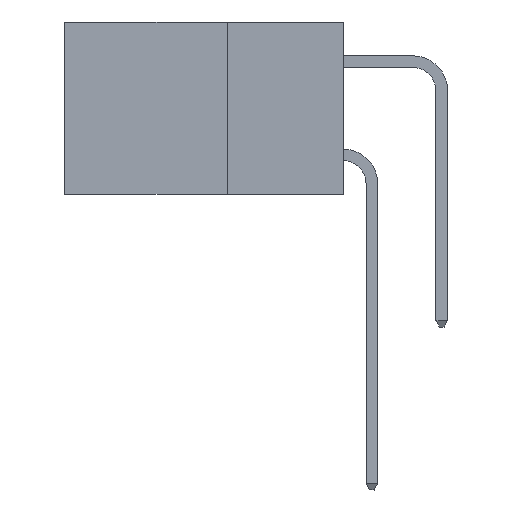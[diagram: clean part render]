
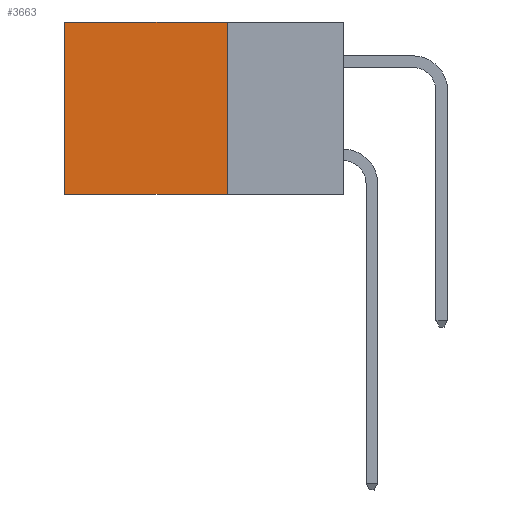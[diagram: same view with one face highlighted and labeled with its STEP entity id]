
A CAD part, left-side view. The second image highlights one B-rep face of the part: STEP entity #3663.
In plain terms, the highlighted planar face has unit normal (-1, 0, 0).
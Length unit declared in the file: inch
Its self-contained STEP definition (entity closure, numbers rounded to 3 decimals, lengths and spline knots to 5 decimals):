
#392 = EDGE_LOOP ( 'NONE', ( #25343, #17288, #13534, #23836 ) ) ;
#621 = CARTESIAN_POINT ( 'NONE',  ( 0.2615, 0.25, 0. ) ) ;
#995 = AXIS2_PLACEMENT_3D ( 'NONE', #5181, #7041, #18379 ) ;
#2786 = CARTESIAN_POINT ( 'NONE',  ( 0.2615, 0.25, -0.37 ) ) ;
#3031 = FACE_OUTER_BOUND ( 'NONE', #392, .T. ) ;
#3663 = ADVANCED_FACE ( 'NONE', ( #3031 ), #9621, .F. ) ;
#5181 = CARTESIAN_POINT ( 'NONE',  ( 0.2615, 0.25, -0.37 ) ) ;
#5223 = DIRECTION ( 'NONE',  ( 0., 1., 0. ) ) ;
#6439 = EDGE_CURVE ( 'NONE', #7073, #13860, #22135, .T. ) ;
#7041 = DIRECTION ( 'NONE',  ( 1., 0., 0. ) ) ;
#7073 = VERTEX_POINT ( 'NONE', #27139 ) ;
#8079 = CARTESIAN_POINT ( 'NONE',  ( 0.2615, 0.25, -0.37 ) ) ;
#9621 = PLANE ( 'NONE',  #995 ) ;
#10214 = CARTESIAN_POINT ( 'NONE',  ( 0.2615, 0.6, -0.37 ) ) ;
#10719 = EDGE_CURVE ( 'NONE', #11330, #28137, #19257, .T. ) ;
#11330 = VERTEX_POINT ( 'NONE', #27355 ) ;
#11357 = LINE ( 'NONE', #621, #17912 ) ;
#11728 = CARTESIAN_POINT ( 'NONE',  ( 0.2615, 0.25, -0.37 ) ) ;
#11998 = EDGE_CURVE ( 'NONE', #13860, #28137, #18979, .T. ) ;
#12691 = VECTOR ( 'NONE', #15079, 39.37008 ) ;
#13534 = ORIENTED_EDGE ( 'NONE', *, *, #6439, .F. ) ;
#13860 = VERTEX_POINT ( 'NONE', #11728 ) ;
#14116 = VECTOR ( 'NONE', #5223, 39.37008 ) ;
#15079 = DIRECTION ( 'NONE',  ( 0., 0., -1. ) ) ;
#17288 = ORIENTED_EDGE ( 'NONE', *, *, #11998, .F. ) ;
#17813 = EDGE_CURVE ( 'NONE', #7073, #11330, #11357, .T. ) ;
#17912 = VECTOR ( 'NONE', #20396, 39.37008 ) ;
#18265 = DIRECTION ( 'NONE',  ( 0., 0., -1. ) ) ;
#18379 = DIRECTION ( 'NONE',  ( 0., 0., -1. ) ) ;
#18979 = LINE ( 'NONE', #8079, #14116 ) ;
#19257 = LINE ( 'NONE', #10214, #12691 ) ;
#20396 = DIRECTION ( 'NONE',  ( 0., 1., 0. ) ) ;
#22135 = LINE ( 'NONE', #2786, #25371 ) ;
#23836 = ORIENTED_EDGE ( 'NONE', *, *, #17813, .T. ) ;
#25010 = CARTESIAN_POINT ( 'NONE',  ( 0.2615, 0.6, -0.37 ) ) ;
#25343 = ORIENTED_EDGE ( 'NONE', *, *, #10719, .T. ) ;
#25371 = VECTOR ( 'NONE', #18265, 39.37008 ) ;
#27139 = CARTESIAN_POINT ( 'NONE',  ( 0.2615, 0.25, 0. ) ) ;
#27355 = CARTESIAN_POINT ( 'NONE',  ( 0.2615, 0.6, 0. ) ) ;
#28137 = VERTEX_POINT ( 'NONE', #25010 ) ;
